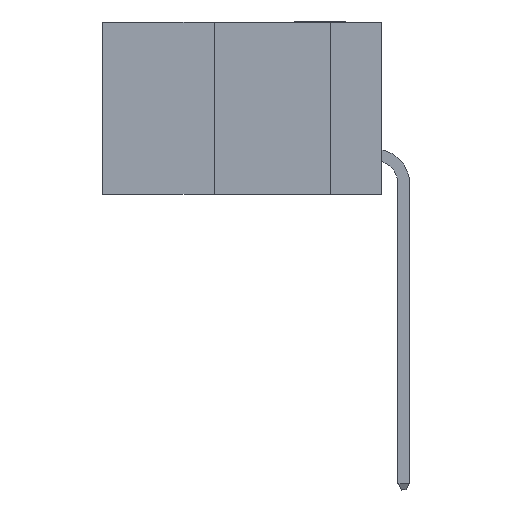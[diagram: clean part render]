
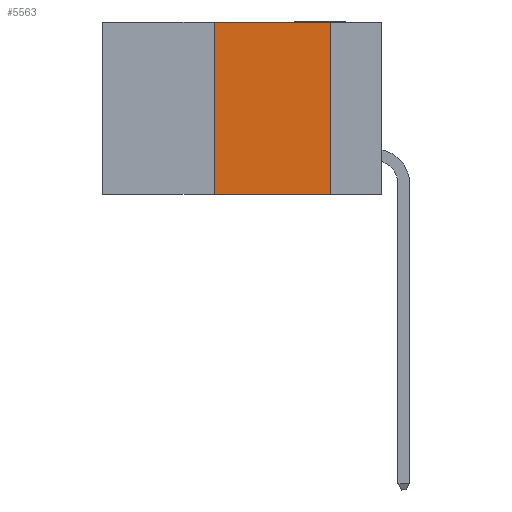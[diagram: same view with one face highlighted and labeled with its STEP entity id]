
A CAD part, left-side view. The second image highlights one B-rep face of the part: STEP entity #5563.
In plain terms, the highlighted planar face has unit normal (-1, 0, 0).
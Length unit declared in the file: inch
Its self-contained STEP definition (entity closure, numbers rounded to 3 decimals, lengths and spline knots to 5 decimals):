
#230 = VERTEX_POINT ( 'NONE', #5434 ) ;
#275 = VECTOR ( 'NONE', #1502, 39.37008 ) ;
#487 = AXIS2_PLACEMENT_3D ( 'NONE', #8741, #4360, #9505 ) ;
#560 = EDGE_CURVE ( 'NONE', #1088, #6310, #7424, .T. ) ;
#1088 = VERTEX_POINT ( 'NONE', #7664 ) ;
#1257 = DIRECTION ( 'NONE',  ( 0., -1., 0. ) ) ;
#1337 = PLANE ( 'NONE',  #487 ) ;
#1502 = DIRECTION ( 'NONE',  ( 0., 0., 1. ) ) ;
#1883 = DIRECTION ( 'NONE',  ( 0., -1., 0. ) ) ;
#1945 = FACE_OUTER_BOUND ( 'NONE', #8578, .T. ) ;
#2500 = VECTOR ( 'NONE', #1883, 39.37008 ) ;
#2668 = CARTESIAN_POINT ( 'NONE',  ( 0., 0.6, 0. ) ) ;
#2782 = CARTESIAN_POINT ( 'NONE',  ( 0., 0.11, -0.37 ) ) ;
#2972 = LINE ( 'NONE', #2668, #2500 ) ;
#2974 = ORIENTED_EDGE ( 'NONE', *, *, #4251, .F. ) ;
#3145 = CARTESIAN_POINT ( 'NONE',  ( 0., 0.11, 0. ) ) ;
#3472 = VECTOR ( 'NONE', #3816, 39.37008 ) ;
#3816 = DIRECTION ( 'NONE',  ( 0., 0., -1. ) ) ;
#4251 = EDGE_CURVE ( 'NONE', #4413, #6310, #5386, .T. ) ;
#4299 = CARTESIAN_POINT ( 'NONE',  ( 0., 0.6, -0.37 ) ) ;
#4360 = DIRECTION ( 'NONE',  ( 1., 0., 0. ) ) ;
#4413 = VERTEX_POINT ( 'NONE', #5568 ) ;
#5128 = VECTOR ( 'NONE', #1257, 39.37008 ) ;
#5386 = LINE ( 'NONE', #3145, #3472 ) ;
#5434 = CARTESIAN_POINT ( 'NONE',  ( 0., 0.36, 0. ) ) ;
#5563 = ADVANCED_FACE ( 'NONE', ( #1945 ), #1337, .F. ) ;
#5568 = CARTESIAN_POINT ( 'NONE',  ( 0., 0.11, 0. ) ) ;
#6184 = LINE ( 'NONE', #6694, #275 ) ;
#6310 = VERTEX_POINT ( 'NONE', #2782 ) ;
#6694 = CARTESIAN_POINT ( 'NONE',  ( 0., 0.36, 0. ) ) ;
#7211 = ORIENTED_EDGE ( 'NONE', *, *, #8971, .F. ) ;
#7424 = LINE ( 'NONE', #4299, #5128 ) ;
#7664 = CARTESIAN_POINT ( 'NONE',  ( 0., 0.36, -0.37 ) ) ;
#8228 = ORIENTED_EDGE ( 'NONE', *, *, #8738, .F. ) ;
#8578 = EDGE_LOOP ( 'NONE', ( #2974, #7211, #8228, #8815 ) ) ;
#8738 = EDGE_CURVE ( 'NONE', #1088, #230, #6184, .T. ) ;
#8741 = CARTESIAN_POINT ( 'NONE',  ( 0., 0.6, 0. ) ) ;
#8815 = ORIENTED_EDGE ( 'NONE', *, *, #560, .T. ) ;
#8971 = EDGE_CURVE ( 'NONE', #230, #4413, #2972, .T. ) ;
#9505 = DIRECTION ( 'NONE',  ( 0., 0., -1. ) ) ;
